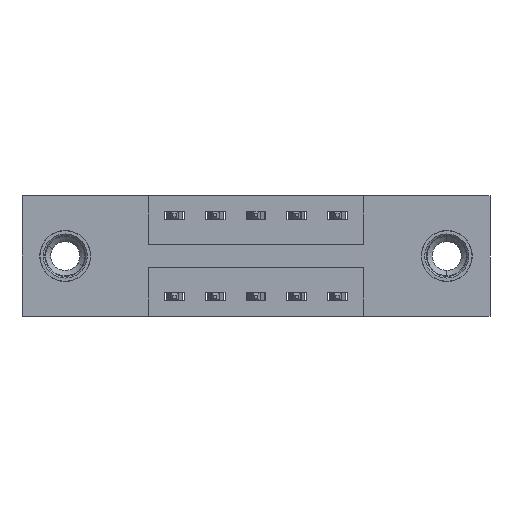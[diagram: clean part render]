
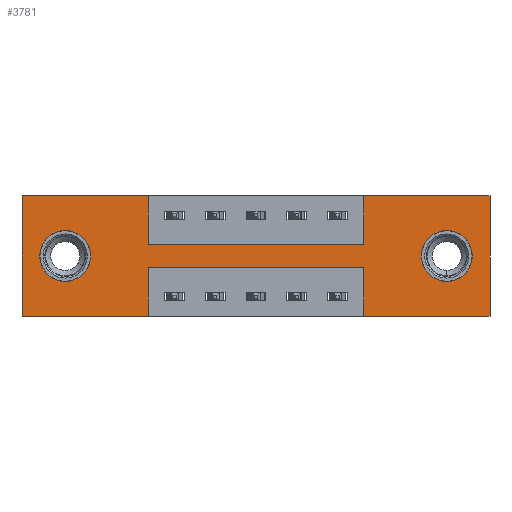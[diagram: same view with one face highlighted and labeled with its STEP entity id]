
A CAD part, front view. The second image highlights one B-rep face of the part: STEP entity #3781.
In plain terms, the highlighted planar face has unit normal (0, -1, 0).
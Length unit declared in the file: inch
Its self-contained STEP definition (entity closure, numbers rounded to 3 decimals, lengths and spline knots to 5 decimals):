
#10 = EDGE_CURVE ( 'NONE', #6729, #977, #8450, .T. ) ;
#11 = CARTESIAN_POINT ( 'NONE',  ( 0.3875, 0., -0.37 ) ) ;
#15 = DIRECTION ( 'NONE',  ( 0., 0., -1. ) ) ;
#74 = ORIENTED_EDGE ( 'NONE', *, *, #1394, .T. ) ;
#134 = CARTESIAN_POINT ( 'NONE',  ( 0.3875, 0., -0.37 ) ) ;
#138 = DIRECTION ( 'NONE',  ( 0., 0., 1. ) ) ;
#143 = LINE ( 'NONE', #8308, #1184 ) ;
#199 = VERTEX_POINT ( 'NONE', #7933 ) ;
#311 = CARTESIAN_POINT ( 'NONE',  ( 0., 0., 0. ) ) ;
#315 = EDGE_CURVE ( 'NONE', #1961, #5409, #6878, .T. ) ;
#325 = ORIENTED_EDGE ( 'NONE', *, *, #6653, .F. ) ;
#331 = VERTEX_POINT ( 'NONE', #1731 ) ;
#440 = EDGE_CURVE ( 'NONE', #2802, #2492, #6643, .T. ) ;
#449 = CIRCLE ( 'NONE', #9445, 0.078 ) ;
#664 = DIRECTION ( 'NONE',  ( 0., 0., -1. ) ) ;
#665 = DIRECTION ( 'NONE',  ( 0., 1., 0. ) ) ;
#675 = CARTESIAN_POINT ( 'NONE',  ( 1.3025, 0., -0.185 ) ) ;
#791 = AXIS2_PLACEMENT_3D ( 'NONE', #4475, #4289, #4288 ) ;
#879 = VERTEX_POINT ( 'NONE', #2047 ) ;
#910 = CARTESIAN_POINT ( 'NONE',  ( 1.0475, 0., 0. ) ) ;
#977 = VERTEX_POINT ( 'NONE', #9405 ) ;
#1051 = CARTESIAN_POINT ( 'NONE',  ( 0., 0., 0. ) ) ;
#1174 = DIRECTION ( 'NONE',  ( 1., 0., 0. ) ) ;
#1184 = VECTOR ( 'NONE', #8337, 39.37008 ) ;
#1233 = AXIS2_PLACEMENT_3D ( 'NONE', #9407, #9371, #5780 ) ;
#1309 = DIRECTION ( 'NONE',  ( 0., 0., 1. ) ) ;
#1394 = EDGE_CURVE ( 'NONE', #3435, #331, #2926, .T. ) ;
#1404 = ORIENTED_EDGE ( 'NONE', *, *, #4157, .F. ) ;
#1447 = ORIENTED_EDGE ( 'NONE', *, *, #315, .F. ) ;
#1505 = DIRECTION ( 'NONE',  ( 0., 0., 1. ) ) ;
#1508 = AXIS2_PLACEMENT_3D ( 'NONE', #6468, #6450, #6437 ) ;
#1569 = ORIENTED_EDGE ( 'NONE', *, *, #5984, .T. ) ;
#1619 = CARTESIAN_POINT ( 'NONE',  ( 1.0475, 0., -0.37 ) ) ;
#1731 = CARTESIAN_POINT ( 'NONE',  ( 1.3025, 0., -0.107 ) ) ;
#1887 = VECTOR ( 'NONE', #5329, 39.37008 ) ;
#1961 = VERTEX_POINT ( 'NONE', #2666 ) ;
#2012 = VECTOR ( 'NONE', #1309, 39.37008 ) ;
#2032 = LINE ( 'NONE', #910, #2012 ) ;
#2047 = CARTESIAN_POINT ( 'NONE',  ( 0.3875, 0., -0.22 ) ) ;
#2161 = VECTOR ( 'NONE', #1505, 39.37008 ) ;
#2234 = DIRECTION ( 'NONE',  ( 1., 0., 0. ) ) ;
#2243 = CARTESIAN_POINT ( 'NONE',  ( 0.1325, 0., -0.107 ) ) ;
#2377 = ORIENTED_EDGE ( 'NONE', *, *, #3090, .F. ) ;
#2394 = LINE ( 'NONE', #1619, #2161 ) ;
#2492 = VERTEX_POINT ( 'NONE', #7624 ) ;
#2516 = VECTOR ( 'NONE', #9263, 39.37008 ) ;
#2617 = LINE ( 'NONE', #9244, #2516 ) ;
#2666 = CARTESIAN_POINT ( 'NONE',  ( 0., 0., 0. ) ) ;
#2802 = VERTEX_POINT ( 'NONE', #4531 ) ;
#2898 = VECTOR ( 'NONE', #15, 39.37008 ) ;
#2926 = CIRCLE ( 'NONE', #1508, 0.078 ) ;
#3006 = VECTOR ( 'NONE', #3375, 39.37008 ) ;
#3062 = CARTESIAN_POINT ( 'NONE',  ( 1.0475, 0., -0.22 ) ) ;
#3090 = EDGE_CURVE ( 'NONE', #199, #1961, #6477, .T. ) ;
#3099 = LINE ( 'NONE', #11, #2898 ) ;
#3106 = LINE ( 'NONE', #3477, #3006 ) ;
#3132 = ORIENTED_EDGE ( 'NONE', *, *, #6840, .F. ) ;
#3234 = LINE ( 'NONE', #5481, #1887 ) ;
#3324 = ORIENTED_EDGE ( 'NONE', *, *, #4702, .T. ) ;
#3375 = DIRECTION ( 'NONE',  ( -1., 0., 0. ) ) ;
#3433 = CARTESIAN_POINT ( 'NONE',  ( 0.3875, 0., 0. ) ) ;
#3435 = VERTEX_POINT ( 'NONE', #8623 ) ;
#3477 = CARTESIAN_POINT ( 'NONE',  ( 0.3875, 0., -0.22 ) ) ;
#3539 = EDGE_LOOP ( 'NONE', ( #8733, #325, #5776, #1404, #5931, #5650, #3132, #3817, #4986, #1447, #2377, #8993 ) ) ;
#3628 = CARTESIAN_POINT ( 'NONE',  ( 1.0475, 0., -0.15 ) ) ;
#3684 = FACE_BOUND ( 'NONE', #6475, .T. ) ;
#3729 = FACE_BOUND ( 'NONE', #9388, .T. ) ;
#3745 = VECTOR ( 'NONE', #4633, 39.37008 ) ;
#3756 = FACE_OUTER_BOUND ( 'NONE', #3539, .T. ) ;
#3764 = EDGE_CURVE ( 'NONE', #2492, #7257, #3800, .T. ) ;
#3781 = ADVANCED_FACE ( 'NONE', ( #3684, #3729, #3756 ), #4427, .T. ) ;
#3800 = LINE ( 'NONE', #4650, #3745 ) ;
#3817 = ORIENTED_EDGE ( 'NONE', *, *, #7070, .F. ) ;
#4103 = EDGE_CURVE ( 'NONE', #879, #9312, #3099, .T. ) ;
#4157 = EDGE_CURVE ( 'NONE', #7257, #4224, #2617, .T. ) ;
#4224 = VERTEX_POINT ( 'NONE', #8849 ) ;
#4288 = DIRECTION ( 'NONE',  ( 0., 0., -1. ) ) ;
#4289 = DIRECTION ( 'NONE',  ( 0., -1., 0. ) ) ;
#4372 = AXIS2_PLACEMENT_3D ( 'NONE', #675, #665, #664 ) ;
#4427 = PLANE ( 'NONE',  #791 ) ;
#4475 = CARTESIAN_POINT ( 'NONE',  ( 0., 0., -0.37 ) ) ;
#4531 = CARTESIAN_POINT ( 'NONE',  ( 1.0475, 0., 0. ) ) ;
#4633 = DIRECTION ( 'NONE',  ( 0., 0., -1. ) ) ;
#4650 = CARTESIAN_POINT ( 'NONE',  ( 1.435, 0., 0. ) ) ;
#4702 = EDGE_CURVE ( 'NONE', #977, #6729, #449, .T. ) ;
#4986 = ORIENTED_EDGE ( 'NONE', *, *, #7411, .F. ) ;
#5041 = EDGE_CURVE ( 'NONE', #9312, #199, #3234, .T. ) ;
#5329 = DIRECTION ( 'NONE',  ( -1., 0., 0. ) ) ;
#5342 = VERTEX_POINT ( 'NONE', #3628 ) ;
#5409 = VERTEX_POINT ( 'NONE', #3433 ) ;
#5481 = CARTESIAN_POINT ( 'NONE',  ( 0., 0., -0.37 ) ) ;
#5527 = VERTEX_POINT ( 'NONE', #3062 ) ;
#5650 = ORIENTED_EDGE ( 'NONE', *, *, #440, .F. ) ;
#5776 = ORIENTED_EDGE ( 'NONE', *, *, #6799, .F. ) ;
#5780 = DIRECTION ( 'NONE',  ( 0., 0., 1. ) ) ;
#5890 = ORIENTED_EDGE ( 'NONE', *, *, #10, .T. ) ;
#5931 = ORIENTED_EDGE ( 'NONE', *, *, #3764, .F. ) ;
#5984 = EDGE_CURVE ( 'NONE', #331, #3435, #7470, .T. ) ;
#6155 = CARTESIAN_POINT ( 'NONE',  ( 0., 0., 0. ) ) ;
#6437 = DIRECTION ( 'NONE',  ( 0., 0., -1. ) ) ;
#6450 = DIRECTION ( 'NONE',  ( 0., 1., 0. ) ) ;
#6463 = VECTOR ( 'NONE', #138, 39.37008 ) ;
#6468 = CARTESIAN_POINT ( 'NONE',  ( 1.3025, 0., -0.185 ) ) ;
#6475 = EDGE_LOOP ( 'NONE', ( #1569, #74 ) ) ;
#6477 = LINE ( 'NONE', #311, #6463 ) ;
#6480 = DIRECTION ( 'NONE',  ( 0., 0., -1. ) ) ;
#6491 = CARTESIAN_POINT ( 'NONE',  ( 0.3875, 0., 0. ) ) ;
#6559 = VECTOR ( 'NONE', #2234, 39.37008 ) ;
#6572 = VECTOR ( 'NONE', #6480, 39.37008 ) ;
#6643 = LINE ( 'NONE', #6155, #6559 ) ;
#6653 = EDGE_CURVE ( 'NONE', #5527, #879, #3106, .T. ) ;
#6729 = VERTEX_POINT ( 'NONE', #2243 ) ;
#6799 = EDGE_CURVE ( 'NONE', #4224, #5527, #2394, .T. ) ;
#6840 = EDGE_CURVE ( 'NONE', #5342, #2802, #2032, .T. ) ;
#6867 = VECTOR ( 'NONE', #1174, 39.37008 ) ;
#6878 = LINE ( 'NONE', #1051, #6867 ) ;
#7070 = EDGE_CURVE ( 'NONE', #9062, #5342, #143, .T. ) ;
#7101 = DIRECTION ( 'NONE',  ( 0., 0., 1. ) ) ;
#7109 = DIRECTION ( 'NONE',  ( 0., 1., 0. ) ) ;
#7118 = CARTESIAN_POINT ( 'NONE',  ( 0.1325, 0., -0.185 ) ) ;
#7257 = VERTEX_POINT ( 'NONE', #7355 ) ;
#7355 = CARTESIAN_POINT ( 'NONE',  ( 1.435, 0., -0.37 ) ) ;
#7411 = EDGE_CURVE ( 'NONE', #5409, #9062, #8163, .T. ) ;
#7470 = CIRCLE ( 'NONE', #4372, 0.078 ) ;
#7624 = CARTESIAN_POINT ( 'NONE',  ( 1.435, 0., 0. ) ) ;
#7933 = CARTESIAN_POINT ( 'NONE',  ( 0., 0., -0.37 ) ) ;
#8109 = CARTESIAN_POINT ( 'NONE',  ( 0.3875, 0., -0.15 ) ) ;
#8163 = LINE ( 'NONE', #6491, #6572 ) ;
#8308 = CARTESIAN_POINT ( 'NONE',  ( 0.3875, 0., -0.15 ) ) ;
#8337 = DIRECTION ( 'NONE',  ( 1., 0., 0. ) ) ;
#8450 = CIRCLE ( 'NONE', #1233, 0.078 ) ;
#8623 = CARTESIAN_POINT ( 'NONE',  ( 1.3025, 0., -0.263 ) ) ;
#8733 = ORIENTED_EDGE ( 'NONE', *, *, #4103, .F. ) ;
#8849 = CARTESIAN_POINT ( 'NONE',  ( 1.0475, 0., -0.37 ) ) ;
#8993 = ORIENTED_EDGE ( 'NONE', *, *, #5041, .F. ) ;
#9062 = VERTEX_POINT ( 'NONE', #8109 ) ;
#9244 = CARTESIAN_POINT ( 'NONE',  ( 0., 0., -0.37 ) ) ;
#9263 = DIRECTION ( 'NONE',  ( -1., 0., 0. ) ) ;
#9312 = VERTEX_POINT ( 'NONE', #134 ) ;
#9371 = DIRECTION ( 'NONE',  ( 0., 1., 0. ) ) ;
#9388 = EDGE_LOOP ( 'NONE', ( #5890, #3324 ) ) ;
#9405 = CARTESIAN_POINT ( 'NONE',  ( 0.1325, 0., -0.263 ) ) ;
#9407 = CARTESIAN_POINT ( 'NONE',  ( 0.1325, 0., -0.185 ) ) ;
#9445 = AXIS2_PLACEMENT_3D ( 'NONE', #7118, #7109, #7101 ) ;
